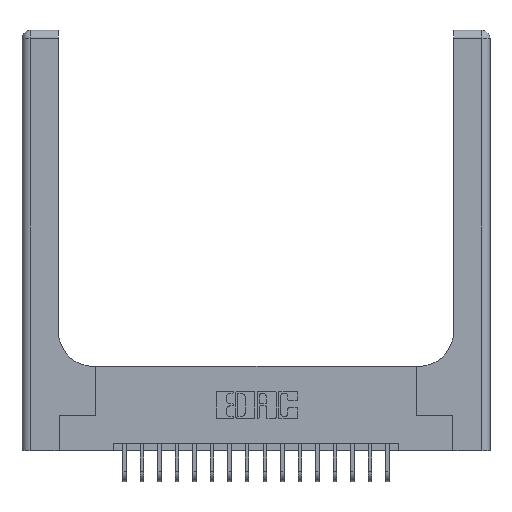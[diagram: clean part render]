
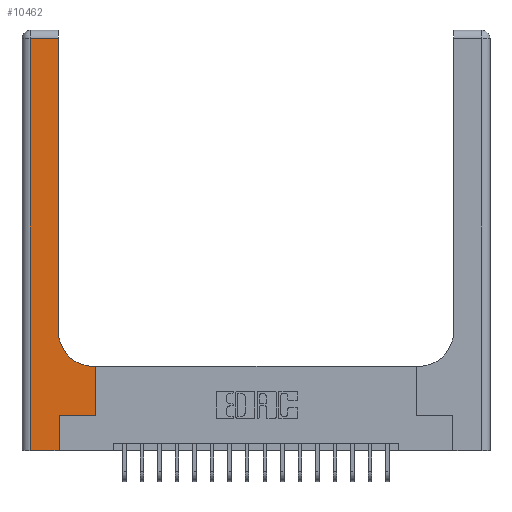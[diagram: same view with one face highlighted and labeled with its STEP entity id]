
A CAD part, top view. The second image highlights one B-rep face of the part: STEP entity #10462.
In plain terms, the highlighted planar face has unit normal (0, 0, 1).
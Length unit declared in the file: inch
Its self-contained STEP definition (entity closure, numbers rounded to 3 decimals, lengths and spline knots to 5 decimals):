
#27 = CARTESIAN_POINT ( 'NONE',  ( 0.06, 0., 0.37 ) ) ;
#85 = ORIENTED_EDGE ( 'NONE', *, *, #17163, .T. ) ;
#104 = AXIS2_PLACEMENT_3D ( 'NONE', #2294, #15463, #7260 ) ;
#109 = LINE ( 'NONE', #6919, #5855 ) ;
#1034 = ORIENTED_EDGE ( 'NONE', *, *, #12754, .T. ) ;
#1328 = LINE ( 'NONE', #15914, #13544 ) ;
#1426 = ORIENTED_EDGE ( 'NONE', *, *, #20935, .T. ) ;
#1828 = AXIS2_PLACEMENT_3D ( 'NONE', #2176, #5418, #1977 ) ;
#1865 = CARTESIAN_POINT ( 'NONE',  ( 0.51, 0.6, 0.37 ) ) ;
#1878 = VECTOR ( 'NONE', #6882, 39.37008 ) ;
#1977 = DIRECTION ( 'NONE',  ( 1., 0., 0. ) ) ;
#2176 = CARTESIAN_POINT ( 'NONE',  ( 0.51, 0.85, 0.37 ) ) ;
#2294 = CARTESIAN_POINT ( 'NONE',  ( 0., 3., 0.37 ) ) ;
#2504 = ORIENTED_EDGE ( 'NONE', *, *, #2702, .T. ) ;
#2702 = EDGE_CURVE ( 'NONE', #8182, #7491, #109, .T. ) ;
#2900 = CARTESIAN_POINT ( 'NONE',  ( 0.528, 0.6, 0.37 ) ) ;
#3141 = VECTOR ( 'NONE', #21349, 39.37008 ) ;
#3283 = ORIENTED_EDGE ( 'NONE', *, *, #16945, .T. ) ;
#3896 = CIRCLE ( 'NONE', #1828, 0.25 ) ;
#4254 = LINE ( 'NONE', #4679, #11146 ) ;
#4364 = DIRECTION ( 'NONE',  ( -1., 0., 0. ) ) ;
#4679 = CARTESIAN_POINT ( 'NONE',  ( 0.26, 0.6, 0.37 ) ) ;
#5298 = DIRECTION ( 'NONE',  ( 0., 1., 0. ) ) ;
#5418 = DIRECTION ( 'NONE',  ( 0., 0., -1. ) ) ;
#5767 = LINE ( 'NONE', #12363, #19218 ) ;
#5855 = VECTOR ( 'NONE', #5298, 39.37008 ) ;
#6065 = LINE ( 'NONE', #21267, #8982 ) ;
#6199 = DIRECTION ( 'NONE',  ( 1., 0., 0. ) ) ;
#6830 = VERTEX_POINT ( 'NONE', #27 ) ;
#6882 = DIRECTION ( 'NONE',  ( -1., 0., 0. ) ) ;
#6919 = CARTESIAN_POINT ( 'NONE',  ( 0.265, 0., 0.37 ) ) ;
#7095 = CARTESIAN_POINT ( 'NONE',  ( 0., 2.94, 0.37 ) ) ;
#7260 = DIRECTION ( 'NONE',  ( -1., 0., 0. ) ) ;
#7349 = EDGE_CURVE ( 'NONE', #14494, #20906, #6065, .T. ) ;
#7385 = ORIENTED_EDGE ( 'NONE', *, *, #7349, .T. ) ;
#7491 = VERTEX_POINT ( 'NONE', #18857 ) ;
#7810 = EDGE_CURVE ( 'NONE', #6830, #8182, #16590, .T. ) ;
#7995 = ORIENTED_EDGE ( 'NONE', *, *, #7810, .T. ) ;
#8182 = VERTEX_POINT ( 'NONE', #20459 ) ;
#8698 = LINE ( 'NONE', #8808, #10931 ) ;
#8808 = CARTESIAN_POINT ( 'NONE',  ( 0.528, 0.25, 0.37 ) ) ;
#8861 = VERTEX_POINT ( 'NONE', #1865 ) ;
#8982 = VECTOR ( 'NONE', #11564, 39.37008 ) ;
#10271 = CARTESIAN_POINT ( 'NONE',  ( 0.06, 2.94, 0.37 ) ) ;
#10462 = ADVANCED_FACE ( 'NONE', ( #18705 ), #10510, .F. ) ;
#10510 = PLANE ( 'NONE',  #104 ) ;
#10931 = VECTOR ( 'NONE', #16999, 39.37008 ) ;
#11146 = VECTOR ( 'NONE', #4364, 39.37008 ) ;
#11564 = DIRECTION ( 'NONE',  ( 0., 1., 0. ) ) ;
#12014 = EDGE_CURVE ( 'NONE', #8861, #14494, #3896, .T. ) ;
#12266 = VERTEX_POINT ( 'NONE', #10271 ) ;
#12363 = CARTESIAN_POINT ( 'NONE',  ( 0.06, 3., 0.37 ) ) ;
#12754 = EDGE_CURVE ( 'NONE', #20906, #12266, #13580, .T. ) ;
#13002 = ORIENTED_EDGE ( 'NONE', *, *, #20907, .T. ) ;
#13522 = CARTESIAN_POINT ( 'NONE',  ( 0.26, 0.85, 0.37 ) ) ;
#13544 = VECTOR ( 'NONE', #6199, 39.37008 ) ;
#13580 = LINE ( 'NONE', #7095, #1878 ) ;
#13741 = ORIENTED_EDGE ( 'NONE', *, *, #12014, .T. ) ;
#14494 = VERTEX_POINT ( 'NONE', #13522 ) ;
#14793 = CARTESIAN_POINT ( 'NONE',  ( 0.528, 0.25, 0.37 ) ) ;
#14916 = VERTEX_POINT ( 'NONE', #14793 ) ;
#15463 = DIRECTION ( 'NONE',  ( 0., 0., -1. ) ) ;
#15914 = CARTESIAN_POINT ( 'NONE',  ( 0.265, 0.25, 0.37 ) ) ;
#16486 = VERTEX_POINT ( 'NONE', #2900 ) ;
#16590 = LINE ( 'NONE', #17784, #3141 ) ;
#16945 = EDGE_CURVE ( 'NONE', #14916, #16486, #8698, .T. ) ;
#16999 = DIRECTION ( 'NONE',  ( 0., 1., 0. ) ) ;
#17163 = EDGE_CURVE ( 'NONE', #12266, #6830, #5767, .T. ) ;
#17319 = DIRECTION ( 'NONE',  ( 0., -1., 0. ) ) ;
#17542 = CARTESIAN_POINT ( 'NONE',  ( 0.26, 2.94, 0.37 ) ) ;
#17784 = CARTESIAN_POINT ( 'NONE',  ( 0., 0., 0.37 ) ) ;
#18705 = FACE_OUTER_BOUND ( 'NONE', #21184, .T. ) ;
#18857 = CARTESIAN_POINT ( 'NONE',  ( 0.265, 0.25, 0.37 ) ) ;
#19218 = VECTOR ( 'NONE', #17319, 39.37008 ) ;
#20459 = CARTESIAN_POINT ( 'NONE',  ( 0.265, 0., 0.37 ) ) ;
#20906 = VERTEX_POINT ( 'NONE', #17542 ) ;
#20907 = EDGE_CURVE ( 'NONE', #16486, #8861, #4254, .T. ) ;
#20935 = EDGE_CURVE ( 'NONE', #7491, #14916, #1328, .T. ) ;
#21184 = EDGE_LOOP ( 'NONE', ( #7385, #1034, #85, #7995, #2504, #1426, #3283, #13002, #13741 ) ) ;
#21267 = CARTESIAN_POINT ( 'NONE',  ( 0.26, 3., 0.37 ) ) ;
#21349 = DIRECTION ( 'NONE',  ( 1., 0., 0. ) ) ;
